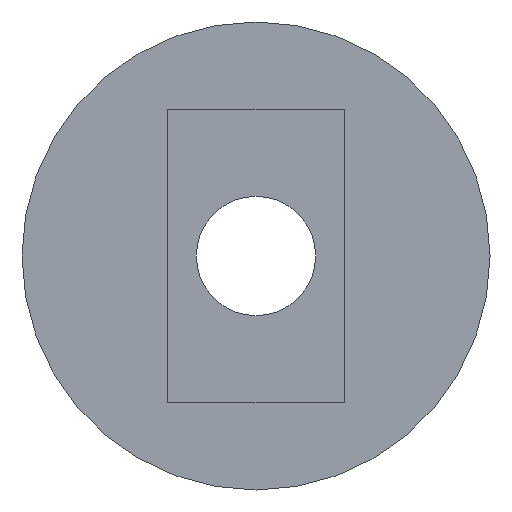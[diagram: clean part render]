
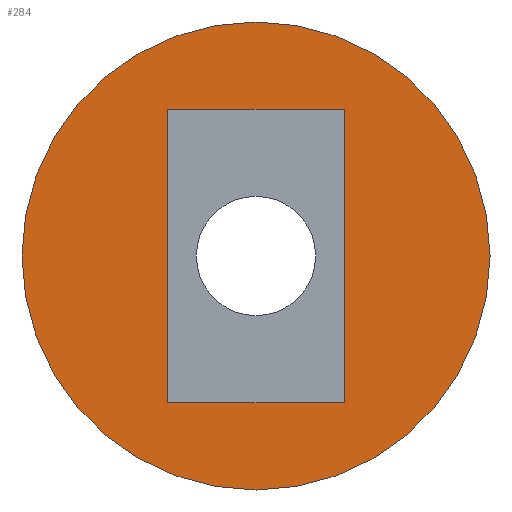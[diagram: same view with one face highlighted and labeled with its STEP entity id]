
A CAD part, front view. The second image highlights one B-rep face of the part: STEP entity #284.
In plain terms, the highlighted planar face has unit normal (0, -1, 0).
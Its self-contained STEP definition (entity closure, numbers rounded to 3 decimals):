
#3 = CARTESIAN_POINT ( 'NONE',  ( 2.29, 1.79, -3.81 ) ) ;
#5 = CARTESIAN_POINT ( 'NONE',  ( -2.29, 1.79, 3.81 ) ) ;
#14 = AXIS2_PLACEMENT_3D ( 'NONE', #339, #87, #383 ) ;
#19 = VECTOR ( 'NONE', #415, 1000. ) ;
#29 = LINE ( 'NONE', #327, #19 ) ;
#58 = ORIENTED_EDGE ( 'NONE', *, *, #332, .T. ) ;
#59 = EDGE_CURVE ( 'NONE', #113, #307, #306, .T. ) ;
#64 = DIRECTION ( 'NONE',  ( 0., 1., 0. ) ) ;
#73 = ORIENTED_EDGE ( 'NONE', *, *, #59, .T. ) ;
#84 = EDGE_CURVE ( 'NONE', #177, #330, #317, .T. ) ;
#87 = DIRECTION ( 'NONE',  ( 0., 1., 0. ) ) ;
#98 = VERTEX_POINT ( 'NONE', #516 ) ;
#109 = VERTEX_POINT ( 'NONE', #229 ) ;
#113 = VERTEX_POINT ( 'NONE', #439 ) ;
#118 = FACE_OUTER_BOUND ( 'NONE', #220, .T. ) ;
#121 = VECTOR ( 'NONE', #194, 1000. ) ;
#142 = DIRECTION ( 'NONE',  ( 0., 0., -1. ) ) ;
#162 = EDGE_CURVE ( 'NONE', #307, #109, #175, .T. ) ;
#175 = LINE ( 'NONE', #480, #121 ) ;
#177 = VERTEX_POINT ( 'NONE', #322 ) ;
#194 = DIRECTION ( 'NONE',  ( -1., 0., 0. ) ) ;
#202 = DIRECTION ( 'NONE',  ( 0., 1., 0. ) ) ;
#220 = EDGE_LOOP ( 'NONE', ( #475, #476 ) ) ;
#229 = CARTESIAN_POINT ( 'NONE',  ( -2.29, 1.79, -3.81 ) ) ;
#275 = EDGE_CURVE ( 'NONE', #109, #98, #29, .T. ) ;
#284 = ADVANCED_FACE ( 'NONE', ( #118, #453 ), #289, .F. ) ;
#289 = PLANE ( 'NONE',  #386 ) ;
#297 = CIRCLE ( 'NONE', #14, 6.085 ) ;
#306 = LINE ( 'NONE', #434, #517 ) ;
#307 = VERTEX_POINT ( 'NONE', #3 ) ;
#315 = CARTESIAN_POINT ( 'NONE',  ( 0., 1.79, 0. ) ) ;
#317 = CIRCLE ( 'NONE', #338, 6.085 ) ;
#322 = CARTESIAN_POINT ( 'NONE',  ( 0., 1.79, 6.085 ) ) ;
#327 = CARTESIAN_POINT ( 'NONE',  ( -2.29, 1.79, -3.81 ) ) ;
#328 = EDGE_LOOP ( 'NONE', ( #58, #73, #500, #505 ) ) ;
#330 = VERTEX_POINT ( 'NONE', #333 ) ;
#332 = EDGE_CURVE ( 'NONE', #98, #113, #420, .T. ) ;
#333 = CARTESIAN_POINT ( 'NONE',  ( 0., 1.79, -6.085 ) ) ;
#338 = AXIS2_PLACEMENT_3D ( 'NONE', #315, #64, #358 ) ;
#339 = CARTESIAN_POINT ( 'NONE',  ( 0., 1.79, 0. ) ) ;
#358 = DIRECTION ( 'NONE',  ( 0., 0., 1. ) ) ;
#375 = CARTESIAN_POINT ( 'NONE',  ( 0., 1.79, 0. ) ) ;
#383 = DIRECTION ( 'NONE',  ( 0., 0., 1. ) ) ;
#386 = AXIS2_PLACEMENT_3D ( 'NONE', #375, #202, #490 ) ;
#389 = EDGE_CURVE ( 'NONE', #330, #177, #297, .T. ) ;
#415 = DIRECTION ( 'NONE',  ( 0., 0., 1. ) ) ;
#419 = DIRECTION ( 'NONE',  ( 1., 0., 0. ) ) ;
#420 = LINE ( 'NONE', #5, #523 ) ;
#434 = CARTESIAN_POINT ( 'NONE',  ( 2.29, 1.79, -3.81 ) ) ;
#439 = CARTESIAN_POINT ( 'NONE',  ( 2.29, 1.79, 3.81 ) ) ;
#453 = FACE_BOUND ( 'NONE', #328, .T. ) ;
#475 = ORIENTED_EDGE ( 'NONE', *, *, #389, .F. ) ;
#476 = ORIENTED_EDGE ( 'NONE', *, *, #84, .F. ) ;
#480 = CARTESIAN_POINT ( 'NONE',  ( -2.29, 1.79, -3.81 ) ) ;
#490 = DIRECTION ( 'NONE',  ( 0., 0., 1. ) ) ;
#500 = ORIENTED_EDGE ( 'NONE', *, *, #162, .T. ) ;
#505 = ORIENTED_EDGE ( 'NONE', *, *, #275, .T. ) ;
#516 = CARTESIAN_POINT ( 'NONE',  ( -2.29, 1.79, 3.81 ) ) ;
#517 = VECTOR ( 'NONE', #142, 1000. ) ;
#523 = VECTOR ( 'NONE', #419, 1000. ) ;
